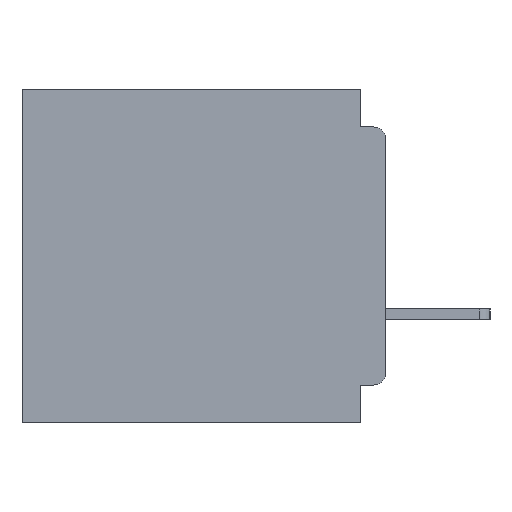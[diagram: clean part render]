
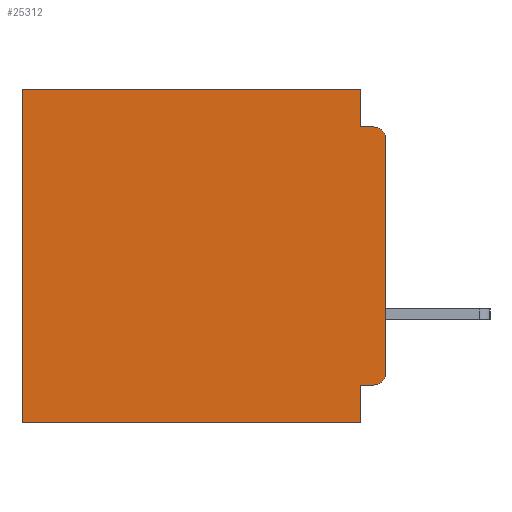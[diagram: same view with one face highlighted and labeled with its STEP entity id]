
A CAD part, left-side view. The second image highlights one B-rep face of the part: STEP entity #25312.
In plain terms, the highlighted planar face has unit normal (-1, 0, 0).
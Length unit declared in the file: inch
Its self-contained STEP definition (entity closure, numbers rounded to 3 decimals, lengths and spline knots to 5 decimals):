
#251 = DIRECTION ( 'NONE',  ( 0., 0., -1. ) ) ;
#787 = LINE ( 'NONE', #25666, #42663 ) ;
#986 = VERTEX_POINT ( 'NONE', #1055 ) ;
#1055 = CARTESIAN_POINT ( 'NONE',  ( 0.3, 0.031, -0.355 ) ) ;
#1557 = CARTESIAN_POINT ( 'NONE',  ( 0.3, 0.015, -0.06 ) ) ;
#2912 = EDGE_CURVE ( 'NONE', #27356, #20725, #26093, .T. ) ;
#3854 = EDGE_CURVE ( 'NONE', #17828, #30374, #12732, .T. ) ;
#4665 = CARTESIAN_POINT ( 'NONE',  ( 0.3, 0.015, -0.34 ) ) ;
#4799 = AXIS2_PLACEMENT_3D ( 'NONE', #1557, #35729, #33560 ) ;
#4962 = EDGE_CURVE ( 'NONE', #26592, #20725, #787, .T. ) ;
#5401 = VECTOR ( 'NONE', #19403, 39.37008 ) ;
#6251 = ORIENTED_EDGE ( 'NONE', *, *, #2912, .T. ) ;
#6649 = EDGE_LOOP ( 'NONE', ( #21599, #6720, #14262, #12111, #32272, #6251, #26451, #10515, #32821, #15852 ) ) ;
#6720 = ORIENTED_EDGE ( 'NONE', *, *, #3854, .T. ) ;
#7267 = CARTESIAN_POINT ( 'NONE',  ( 0.3, 0., 0. ) ) ;
#7413 = DIRECTION ( 'NONE',  ( 0., 1., 0. ) ) ;
#7605 = EDGE_CURVE ( 'NONE', #17828, #18129, #15127, .T. ) ;
#8084 = LINE ( 'NONE', #39411, #29326 ) ;
#8098 = LINE ( 'NONE', #15674, #33038 ) ;
#8130 = DIRECTION ( 'NONE',  ( 0., 0., -1. ) ) ;
#8392 = CARTESIAN_POINT ( 'NONE',  ( 0.3, 0.031, -0.045 ) ) ;
#8430 = EDGE_CURVE ( 'NONE', #32739, #986, #8098, .T. ) ;
#10148 = PLANE ( 'NONE',  #36983 ) ;
#10441 = CARTESIAN_POINT ( 'NONE',  ( 0.3, 0.031, -0.4 ) ) ;
#10515 = ORIENTED_EDGE ( 'NONE', *, *, #19515, .F. ) ;
#12111 = ORIENTED_EDGE ( 'NONE', *, *, #21782, .F. ) ;
#12732 = CIRCLE ( 'NONE', #4799, 0.015 ) ;
#14262 = ORIENTED_EDGE ( 'NONE', *, *, #31215, .F. ) ;
#15127 = LINE ( 'NONE', #35343, #23028 ) ;
#15393 = DIRECTION ( 'NONE',  ( 0., 1., 0. ) ) ;
#15674 = CARTESIAN_POINT ( 'NONE',  ( 0.3, 0., -0.355 ) ) ;
#15852 = ORIENTED_EDGE ( 'NONE', *, *, #36553, .T. ) ;
#16213 = CARTESIAN_POINT ( 'NONE',  ( 0.3, 0.437, -0.4 ) ) ;
#16971 = CARTESIAN_POINT ( 'NONE',  ( 0.3, 0.031, 0. ) ) ;
#17025 = CARTESIAN_POINT ( 'NONE',  ( 0.3, 0., -0.4 ) ) ;
#17104 = VECTOR ( 'NONE', #30475, 39.37008 ) ;
#17828 = VERTEX_POINT ( 'NONE', #35372 ) ;
#18129 = VERTEX_POINT ( 'NONE', #43485 ) ;
#18964 = VECTOR ( 'NONE', #251, 39.37008 ) ;
#19223 = DIRECTION ( 'NONE',  ( 0., -1., 0. ) ) ;
#19403 = DIRECTION ( 'NONE',  ( 0., 0., -1. ) ) ;
#19515 = EDGE_CURVE ( 'NONE', #986, #26592, #27980, .T. ) ;
#20434 = DIRECTION ( 'NONE',  ( 0., 0., -1. ) ) ;
#20725 = VERTEX_POINT ( 'NONE', #16213 ) ;
#20819 = CARTESIAN_POINT ( 'NONE',  ( 0.3, 0.031, -0.4 ) ) ;
#21599 = ORIENTED_EDGE ( 'NONE', *, *, #7605, .F. ) ;
#21782 = EDGE_CURVE ( 'NONE', #25919, #30610, #32514, .T. ) ;
#22771 = CARTESIAN_POINT ( 'NONE',  ( 0.3, 0.031, 0. ) ) ;
#23028 = VECTOR ( 'NONE', #34733, 39.37008 ) ;
#25312 = ADVANCED_FACE ( 'NONE', ( #43436 ), #10148, .F. ) ;
#25497 = CARTESIAN_POINT ( 'NONE',  ( 0.3, 0.437, 0. ) ) ;
#25666 = CARTESIAN_POINT ( 'NONE',  ( 0.3, 0., -0.4 ) ) ;
#25919 = VERTEX_POINT ( 'NONE', #16971 ) ;
#26093 = LINE ( 'NONE', #43331, #17104 ) ;
#26451 = ORIENTED_EDGE ( 'NONE', *, *, #4962, .F. ) ;
#26592 = VERTEX_POINT ( 'NONE', #20819 ) ;
#27356 = VERTEX_POINT ( 'NONE', #25497 ) ;
#27980 = LINE ( 'NONE', #10441, #18964 ) ;
#28460 = DIRECTION ( 'NONE',  ( -1., 0., 0. ) ) ;
#29326 = VECTOR ( 'NONE', #19223, 39.37008 ) ;
#29649 = DIRECTION ( 'NONE',  ( 0., 1., 0. ) ) ;
#30148 = VECTOR ( 'NONE', #7413, 39.37008 ) ;
#30374 = VERTEX_POINT ( 'NONE', #41231 ) ;
#30475 = DIRECTION ( 'NONE',  ( 0., 0., -1. ) ) ;
#30610 = VERTEX_POINT ( 'NONE', #8392 ) ;
#31215 = EDGE_CURVE ( 'NONE', #30610, #30374, #8084, .T. ) ;
#32272 = ORIENTED_EDGE ( 'NONE', *, *, #39938, .T. ) ;
#32514 = LINE ( 'NONE', #22771, #5401 ) ;
#32739 = VERTEX_POINT ( 'NONE', #40873 ) ;
#32821 = ORIENTED_EDGE ( 'NONE', *, *, #8430, .F. ) ;
#33038 = VECTOR ( 'NONE', #15393, 39.37008 ) ;
#33560 = DIRECTION ( 'NONE',  ( 0., 0., -1. ) ) ;
#34733 = DIRECTION ( 'NONE',  ( 0., 0., -1. ) ) ;
#35343 = CARTESIAN_POINT ( 'NONE',  ( 0.3, 0., -0.4 ) ) ;
#35372 = CARTESIAN_POINT ( 'NONE',  ( 0.3, 0., -0.06 ) ) ;
#35729 = DIRECTION ( 'NONE',  ( -1., 0., 0. ) ) ;
#36553 = EDGE_CURVE ( 'NONE', #32739, #18129, #37634, .T. ) ;
#36983 = AXIS2_PLACEMENT_3D ( 'NONE', #17025, #40590, #20434 ) ;
#37634 = CIRCLE ( 'NONE', #41116, 0.015 ) ;
#39082 = LINE ( 'NONE', #7267, #30148 ) ;
#39411 = CARTESIAN_POINT ( 'NONE',  ( 0.3, 0., -0.045 ) ) ;
#39938 = EDGE_CURVE ( 'NONE', #25919, #27356, #39082, .T. ) ;
#40590 = DIRECTION ( 'NONE',  ( 1., 0., 0. ) ) ;
#40873 = CARTESIAN_POINT ( 'NONE',  ( 0.3, 0.015, -0.355 ) ) ;
#41116 = AXIS2_PLACEMENT_3D ( 'NONE', #4665, #28460, #8130 ) ;
#41231 = CARTESIAN_POINT ( 'NONE',  ( 0.3, 0.015, -0.045 ) ) ;
#42663 = VECTOR ( 'NONE', #29649, 39.37008 ) ;
#43331 = CARTESIAN_POINT ( 'NONE',  ( 0.3, 0.437, -0.4 ) ) ;
#43436 = FACE_OUTER_BOUND ( 'NONE', #6649, .T. ) ;
#43485 = CARTESIAN_POINT ( 'NONE',  ( 0.3, 0., -0.34 ) ) ;
